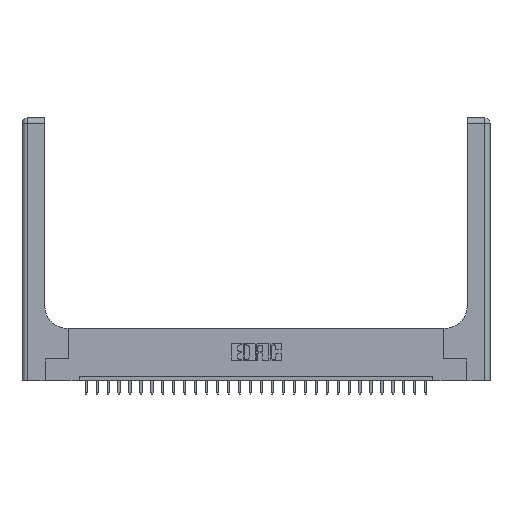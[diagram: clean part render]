
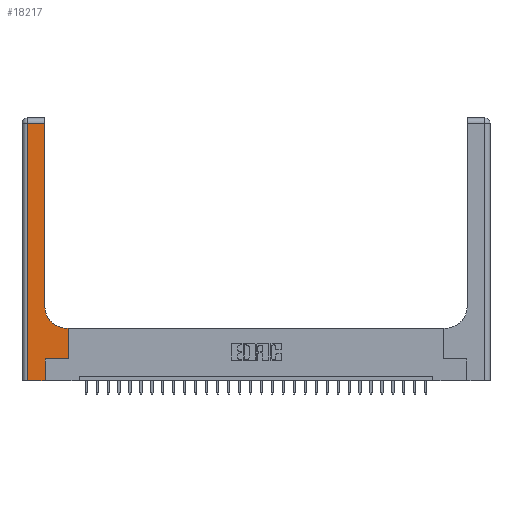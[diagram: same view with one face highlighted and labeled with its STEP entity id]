
A CAD part, top view. The second image highlights one B-rep face of the part: STEP entity #18217.
In plain terms, the highlighted planar face has unit normal (0, 0, 1).
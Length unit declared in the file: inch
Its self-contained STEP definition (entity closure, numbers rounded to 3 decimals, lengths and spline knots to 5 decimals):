
#678 = ORIENTED_EDGE ( 'NONE', *, *, #21907, .T. ) ;
#952 = VERTEX_POINT ( 'NONE', #19235 ) ;
#1337 = CARTESIAN_POINT ( 'NONE',  ( 0.26, 3., 0.37 ) ) ;
#1578 = CARTESIAN_POINT ( 'NONE',  ( 0.26, 0.6, 0.37 ) ) ;
#1973 = LINE ( 'NONE', #1578, #14918 ) ;
#2305 = EDGE_CURVE ( 'NONE', #14495, #7086, #23883, .T. ) ;
#2602 = VECTOR ( 'NONE', #10341, 39.37008 ) ;
#2678 = VERTEX_POINT ( 'NONE', #25248 ) ;
#2706 = CARTESIAN_POINT ( 'NONE',  ( 0., 0., 0.37 ) ) ;
#2835 = DIRECTION ( 'NONE',  ( 1., 0., 0. ) ) ;
#3425 = CARTESIAN_POINT ( 'NONE',  ( 0.265, 0.25, 0.37 ) ) ;
#3441 = EDGE_CURVE ( 'NONE', #11014, #2678, #22467, .T. ) ;
#3865 = VECTOR ( 'NONE', #15903, 39.37008 ) ;
#3871 = DIRECTION ( 'NONE',  ( 0., 1., 0. ) ) ;
#4162 = LINE ( 'NONE', #12441, #9811 ) ;
#4196 = ORIENTED_EDGE ( 'NONE', *, *, #3441, .T. ) ;
#4364 = VECTOR ( 'NONE', #3871, 39.37008 ) ;
#5161 = ORIENTED_EDGE ( 'NONE', *, *, #6776, .T. ) ;
#5285 = CARTESIAN_POINT ( 'NONE',  ( 0.528, 0.25, 0.37 ) ) ;
#5498 = LINE ( 'NONE', #12381, #2602 ) ;
#5599 = AXIS2_PLACEMENT_3D ( 'NONE', #24602, #26645, #13626 ) ;
#6726 = ORIENTED_EDGE ( 'NONE', *, *, #2305, .T. ) ;
#6776 = EDGE_CURVE ( 'NONE', #11392, #11468, #5498, .T. ) ;
#7086 = VERTEX_POINT ( 'NONE', #15626 ) ;
#7437 = VECTOR ( 'NONE', #15728, 39.37008 ) ;
#7620 = LINE ( 'NONE', #3425, #3865 ) ;
#8220 = DIRECTION ( 'NONE',  ( 0., 0., -1. ) ) ;
#9074 = CARTESIAN_POINT ( 'NONE',  ( 0.06, 2.94, 0.37 ) ) ;
#9529 = AXIS2_PLACEMENT_3D ( 'NONE', #26690, #8220, #16244 ) ;
#9811 = VECTOR ( 'NONE', #20466, 39.37008 ) ;
#10113 = CARTESIAN_POINT ( 'NONE',  ( 0.265, 0., 0.37 ) ) ;
#10133 = CARTESIAN_POINT ( 'NONE',  ( 0.06, 0., 0.37 ) ) ;
#10341 = DIRECTION ( 'NONE',  ( 0., -1., 0. ) ) ;
#11014 = VERTEX_POINT ( 'NONE', #18731 ) ;
#11254 = CIRCLE ( 'NONE', #9529, 0.25 ) ;
#11392 = VERTEX_POINT ( 'NONE', #9074 ) ;
#11468 = VERTEX_POINT ( 'NONE', #10133 ) ;
#11708 = VERTEX_POINT ( 'NONE', #15282 ) ;
#12076 = ORIENTED_EDGE ( 'NONE', *, *, #16767, .T. ) ;
#12250 = CARTESIAN_POINT ( 'NONE',  ( 0.26, 2.94, 0.37 ) ) ;
#12303 = DIRECTION ( 'NONE',  ( -1., 0., 0. ) ) ;
#12381 = CARTESIAN_POINT ( 'NONE',  ( 0.06, 3., 0.37 ) ) ;
#12441 = CARTESIAN_POINT ( 'NONE',  ( 0., 2.94, 0.37 ) ) ;
#12458 = ORIENTED_EDGE ( 'NONE', *, *, #23267, .T. ) ;
#12822 = EDGE_CURVE ( 'NONE', #13640, #11392, #4162, .T. ) ;
#13626 = DIRECTION ( 'NONE',  ( -1., 0., 0. ) ) ;
#13640 = VERTEX_POINT ( 'NONE', #12250 ) ;
#14025 = PLANE ( 'NONE',  #5599 ) ;
#14146 = FACE_OUTER_BOUND ( 'NONE', #23456, .T. ) ;
#14207 = DIRECTION ( 'NONE',  ( 0., 1., 0. ) ) ;
#14409 = VECTOR ( 'NONE', #14207, 39.37008 ) ;
#14495 = VERTEX_POINT ( 'NONE', #21759 ) ;
#14918 = VECTOR ( 'NONE', #12303, 39.37008 ) ;
#15282 = CARTESIAN_POINT ( 'NONE',  ( 0.51, 0.6, 0.37 ) ) ;
#15626 = CARTESIAN_POINT ( 'NONE',  ( 0.528, 0.6, 0.37 ) ) ;
#15728 = DIRECTION ( 'NONE',  ( 0., 1., 0. ) ) ;
#15903 = DIRECTION ( 'NONE',  ( 1., 0., 0. ) ) ;
#16244 = DIRECTION ( 'NONE',  ( 1., 0., 0. ) ) ;
#16493 = VECTOR ( 'NONE', #2835, 39.37008 ) ;
#16767 = EDGE_CURVE ( 'NONE', #11708, #952, #11254, .T. ) ;
#17555 = EDGE_CURVE ( 'NONE', #2678, #14495, #7620, .T. ) ;
#18217 = ADVANCED_FACE ( 'NONE', ( #14146 ), #14025, .F. ) ;
#18731 = CARTESIAN_POINT ( 'NONE',  ( 0.265, 0., 0.37 ) ) ;
#19235 = CARTESIAN_POINT ( 'NONE',  ( 0.26, 0.85, 0.37 ) ) ;
#19397 = EDGE_CURVE ( 'NONE', #11468, #11014, #21311, .T. ) ;
#19944 = LINE ( 'NONE', #1337, #14409 ) ;
#20466 = DIRECTION ( 'NONE',  ( -1., 0., 0. ) ) ;
#21311 = LINE ( 'NONE', #2706, #16493 ) ;
#21759 = CARTESIAN_POINT ( 'NONE',  ( 0.528, 0.25, 0.37 ) ) ;
#21907 = EDGE_CURVE ( 'NONE', #952, #13640, #19944, .T. ) ;
#22321 = ORIENTED_EDGE ( 'NONE', *, *, #19397, .T. ) ;
#22467 = LINE ( 'NONE', #10113, #4364 ) ;
#23135 = ORIENTED_EDGE ( 'NONE', *, *, #12822, .T. ) ;
#23267 = EDGE_CURVE ( 'NONE', #7086, #11708, #1973, .T. ) ;
#23456 = EDGE_LOOP ( 'NONE', ( #678, #23135, #5161, #22321, #4196, #26542, #6726, #12458, #12076 ) ) ;
#23883 = LINE ( 'NONE', #5285, #7437 ) ;
#24602 = CARTESIAN_POINT ( 'NONE',  ( 0., 3., 0.37 ) ) ;
#25248 = CARTESIAN_POINT ( 'NONE',  ( 0.265, 0.25, 0.37 ) ) ;
#26542 = ORIENTED_EDGE ( 'NONE', *, *, #17555, .T. ) ;
#26645 = DIRECTION ( 'NONE',  ( 0., 0., -1. ) ) ;
#26690 = CARTESIAN_POINT ( 'NONE',  ( 0.51, 0.85, 0.37 ) ) ;
